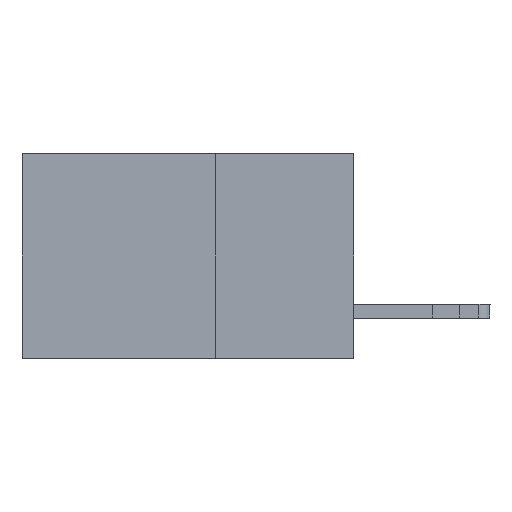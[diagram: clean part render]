
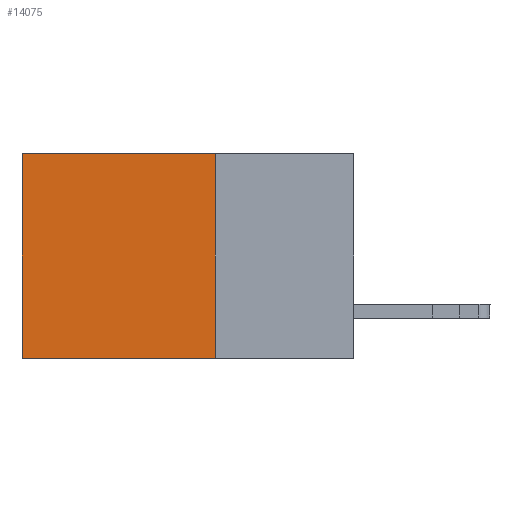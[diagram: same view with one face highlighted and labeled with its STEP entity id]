
A CAD part, left-side view. The second image highlights one B-rep face of the part: STEP entity #14075.
In plain terms, the highlighted planar face has unit normal (-1, 0, 0).
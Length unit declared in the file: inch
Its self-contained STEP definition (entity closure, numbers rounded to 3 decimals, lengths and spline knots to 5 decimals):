
#98 = EDGE_CURVE ( 'NONE', #14456, #13779, #1049, .T. ) ;
#500 = VECTOR ( 'NONE', #12613, 39.37008 ) ;
#574 = CARTESIAN_POINT ( 'NONE',  ( 0.2875, 0.25, -0.37 ) ) ;
#885 = VECTOR ( 'NONE', #1598, 39.37008 ) ;
#1049 = LINE ( 'NONE', #2332, #7396 ) ;
#1463 = ORIENTED_EDGE ( 'NONE', *, *, #13637, .T. ) ;
#1598 = DIRECTION ( 'NONE',  ( 0., 1., 0. ) ) ;
#2332 = CARTESIAN_POINT ( 'NONE',  ( 0.2875, 0.25, 0. ) ) ;
#2558 = VECTOR ( 'NONE', #7313, 39.37008 ) ;
#3536 = DIRECTION ( 'NONE',  ( 0., 0., -1. ) ) ;
#4312 = CARTESIAN_POINT ( 'NONE',  ( 0.2875, 0.25, 0. ) ) ;
#4656 = EDGE_CURVE ( 'NONE', #13779, #13965, #13939, .T. ) ;
#4770 = FACE_OUTER_BOUND ( 'NONE', #10771, .T. ) ;
#5792 = PLANE ( 'NONE',  #14796 ) ;
#5844 = DIRECTION ( 'NONE',  ( 1., 0., 0. ) ) ;
#5914 = CARTESIAN_POINT ( 'NONE',  ( 0.2875, 0.25, -0.37 ) ) ;
#6469 = LINE ( 'NONE', #4312, #500 ) ;
#6682 = ORIENTED_EDGE ( 'NONE', *, *, #98, .F. ) ;
#7313 = DIRECTION ( 'NONE',  ( 0., 0., -1. ) ) ;
#7390 = LINE ( 'NONE', #13267, #2558 ) ;
#7396 = VECTOR ( 'NONE', #3536, 39.37008 ) ;
#8593 = ORIENTED_EDGE ( 'NONE', *, *, #13542, .T. ) ;
#9181 = CARTESIAN_POINT ( 'NONE',  ( 0.2875, 0.6, 0. ) ) ;
#9287 = CARTESIAN_POINT ( 'NONE',  ( 0.2875, 0.25, 0. ) ) ;
#10731 = ORIENTED_EDGE ( 'NONE', *, *, #4656, .F. ) ;
#10771 = EDGE_LOOP ( 'NONE', ( #1463, #10731, #6682, #8593 ) ) ;
#11216 = CARTESIAN_POINT ( 'NONE',  ( 0.2875, 0.6, -0.37 ) ) ;
#12613 = DIRECTION ( 'NONE',  ( 0., 1., 0. ) ) ;
#12973 = CARTESIAN_POINT ( 'NONE',  ( 0.2875, 0.25, 0. ) ) ;
#13041 = DIRECTION ( 'NONE',  ( 0., 0., -1. ) ) ;
#13267 = CARTESIAN_POINT ( 'NONE',  ( 0.2875, 0.6, 0. ) ) ;
#13542 = EDGE_CURVE ( 'NONE', #14456, #14421, #6469, .T. ) ;
#13637 = EDGE_CURVE ( 'NONE', #14421, #13965, #7390, .T. ) ;
#13779 = VERTEX_POINT ( 'NONE', #5914 ) ;
#13939 = LINE ( 'NONE', #574, #885 ) ;
#13965 = VERTEX_POINT ( 'NONE', #11216 ) ;
#14075 = ADVANCED_FACE ( 'NONE', ( #4770 ), #5792, .F. ) ;
#14421 = VERTEX_POINT ( 'NONE', #9181 ) ;
#14456 = VERTEX_POINT ( 'NONE', #9287 ) ;
#14796 = AXIS2_PLACEMENT_3D ( 'NONE', #12973, #5844, #13041 ) ;
